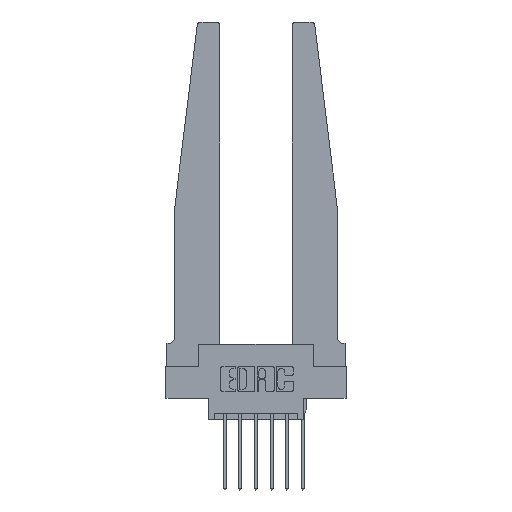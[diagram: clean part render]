
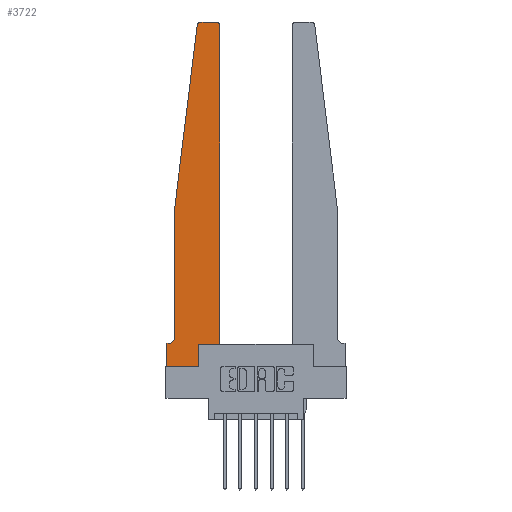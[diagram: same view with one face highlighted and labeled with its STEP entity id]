
A CAD part, top view. The second image highlights one B-rep face of the part: STEP entity #3722.
In plain terms, the highlighted planar face has unit normal (0, 0, 1).
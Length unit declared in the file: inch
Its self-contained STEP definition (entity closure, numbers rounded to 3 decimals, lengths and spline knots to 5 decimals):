
#39 = DIRECTION ( 'NONE',  ( 0., 1., 0. ) ) ;
#136 = EDGE_CURVE ( 'NONE', #623, #9087, #9557, .T. ) ;
#144 = CARTESIAN_POINT ( 'NONE',  ( 0.24675, 2.72367, 0.37 ) ) ;
#162 = VECTOR ( 'NONE', #1716, 39.37008 ) ;
#207 = VECTOR ( 'NONE', #12108, 39.37008 ) ;
#254 = ORIENTED_EDGE ( 'NONE', *, *, #5179, .T. ) ;
#458 = ORIENTED_EDGE ( 'NONE', *, *, #8291, .T. ) ;
#574 = CARTESIAN_POINT ( 'NONE',  ( 0.065, 0.1875, 0.37 ) ) ;
#623 = VERTEX_POINT ( 'NONE', #9569 ) ;
#667 = CARTESIAN_POINT ( 'NONE',  ( 0.425, 0.18, 0.37 ) ) ;
#801 = CARTESIAN_POINT ( 'NONE',  ( 0.065, 1.25, 0.37 ) ) ;
#825 = DIRECTION ( 'NONE',  ( -0.122, -0.992, 0. ) ) ;
#870 = VERTEX_POINT ( 'NONE', #7505 ) ;
#962 = VERTEX_POINT ( 'NONE', #6687 ) ;
#1385 = VECTOR ( 'NONE', #11388, 39.37008 ) ;
#1552 = VERTEX_POINT ( 'NONE', #5206 ) ;
#1575 = CARTESIAN_POINT ( 'NONE',  ( 0.25, 2.75, 0.37 ) ) ;
#1716 = DIRECTION ( 'NONE',  ( 1., 0., 0. ) ) ;
#1934 = LINE ( 'NONE', #9329, #2106 ) ;
#2003 = CIRCLE ( 'NONE', #2866, 0.03 ) ;
#2106 = VECTOR ( 'NONE', #825, 39.37008 ) ;
#2564 = VECTOR ( 'NONE', #4775, 39.37008 ) ;
#2747 = DIRECTION ( 'NONE',  ( 0., 1., 0. ) ) ;
#2781 = AXIS2_PLACEMENT_3D ( 'NONE', #12339, #7245, #10141 ) ;
#2866 = AXIS2_PLACEMENT_3D ( 'NONE', #13142, #8946, #3664 ) ;
#3076 = LINE ( 'NONE', #6185, #162 ) ;
#3124 = CARTESIAN_POINT ( 'NONE',  ( 0.2605, 0.18, 0.37 ) ) ;
#3157 = VERTEX_POINT ( 'NONE', #144 ) ;
#3275 = ORIENTED_EDGE ( 'NONE', *, *, #11091, .T. ) ;
#3395 = VERTEX_POINT ( 'NONE', #9115 ) ;
#3466 = VERTEX_POINT ( 'NONE', #13535 ) ;
#3613 = DIRECTION ( 'NONE',  ( 1., 0., 0. ) ) ;
#3664 = DIRECTION ( 'NONE',  ( 1., 0., 0. ) ) ;
#3722 = ADVANCED_FACE ( 'NONE', ( #5552 ), #6763, .T. ) ;
#3749 = LINE ( 'NONE', #1575, #207 ) ;
#3844 = ORIENTED_EDGE ( 'NONE', *, *, #9715, .T. ) ;
#3959 = ORIENTED_EDGE ( 'NONE', *, *, #136, .T. ) ;
#4170 = ORIENTED_EDGE ( 'NONE', *, *, #6065, .T. ) ;
#4281 = CARTESIAN_POINT ( 'NONE',  ( 0., 0., 0.37 ) ) ;
#4596 = VECTOR ( 'NONE', #39, 39.37008 ) ;
#4775 = DIRECTION ( 'NONE',  ( -1., 0., 0. ) ) ;
#4796 = VERTEX_POINT ( 'NONE', #13323 ) ;
#5005 = DIRECTION ( 'NONE',  ( 0., -1., 0. ) ) ;
#5108 = EDGE_CURVE ( 'NONE', #3466, #10451, #3076, .T. ) ;
#5126 = EDGE_CURVE ( 'NONE', #962, #3395, #13591, .T. ) ;
#5179 = EDGE_CURVE ( 'NONE', #870, #1552, #8766, .T. ) ;
#5206 = CARTESIAN_POINT ( 'NONE',  ( 0.395, 2.75, 0.37 ) ) ;
#5508 = CARTESIAN_POINT ( 'NONE',  ( 0.425, 0.18, 0.37 ) ) ;
#5552 = FACE_OUTER_BOUND ( 'NONE', #10927, .T. ) ;
#5947 = VECTOR ( 'NONE', #11694, 39.37008 ) ;
#6065 = EDGE_CURVE ( 'NONE', #3395, #11338, #9866, .T. ) ;
#6103 = VECTOR ( 'NONE', #5005, 39.37008 ) ;
#6185 = CARTESIAN_POINT ( 'NONE',  ( 0.425, 0.18, 0.37 ) ) ;
#6453 = CARTESIAN_POINT ( 'NONE',  ( 0.015, 0.1875, 0.37 ) ) ;
#6575 = EDGE_CURVE ( 'NONE', #11338, #623, #6877, .T. ) ;
#6599 = ORIENTED_EDGE ( 'NONE', *, *, #6575, .T. ) ;
#6687 = CARTESIAN_POINT ( 'NONE',  ( 0.065, 1.25, 0.37 ) ) ;
#6760 = DIRECTION ( 'NONE',  ( -1., 0., 0. ) ) ;
#6763 = PLANE ( 'NONE',  #11525 ) ;
#6877 = LINE ( 'NONE', #574, #2564 ) ;
#6888 = VERTEX_POINT ( 'NONE', #11595 ) ;
#6959 = LINE ( 'NONE', #667, #4596 ) ;
#7245 = DIRECTION ( 'NONE',  ( 0., 0., 1. ) ) ;
#7371 = LINE ( 'NONE', #3124, #7919 ) ;
#7505 = CARTESIAN_POINT ( 'NONE',  ( 0.425, 2.72, 0.37 ) ) ;
#7919 = VECTOR ( 'NONE', #2747, 39.37008 ) ;
#7932 = CARTESIAN_POINT ( 'NONE',  ( 0.015, 0.2375, 0.37 ) ) ;
#8291 = EDGE_CURVE ( 'NONE', #4796, #3466, #7371, .T. ) ;
#8465 = ORIENTED_EDGE ( 'NONE', *, *, #9701, .T. ) ;
#8557 = ORIENTED_EDGE ( 'NONE', *, *, #5126, .T. ) ;
#8766 = CIRCLE ( 'NONE', #2781, 0.03 ) ;
#8835 = DIRECTION ( 'NONE',  ( 0., 0., -1. ) ) ;
#8839 = CARTESIAN_POINT ( 'NONE',  ( 0., 0.1875, 0.37 ) ) ;
#8946 = DIRECTION ( 'NONE',  ( 0., 0., 1. ) ) ;
#9087 = VERTEX_POINT ( 'NONE', #10060 ) ;
#9115 = CARTESIAN_POINT ( 'NONE',  ( 0.065, 0.2375, 0.37 ) ) ;
#9329 = CARTESIAN_POINT ( 'NONE',  ( 0.065, 1.25, 0.37 ) ) ;
#9557 = LINE ( 'NONE', #4281, #1385 ) ;
#9569 = CARTESIAN_POINT ( 'NONE',  ( 0., 0.1875, 0.37 ) ) ;
#9701 = EDGE_CURVE ( 'NONE', #1552, #6888, #3749, .T. ) ;
#9715 = EDGE_CURVE ( 'NONE', #10451, #870, #6959, .T. ) ;
#9866 = CIRCLE ( 'NONE', #12920, 0.05 ) ;
#10060 = CARTESIAN_POINT ( 'NONE',  ( 0., 0., 0.37 ) ) ;
#10141 = DIRECTION ( 'NONE',  ( 1., 0., 0. ) ) ;
#10451 = VERTEX_POINT ( 'NONE', #5508 ) ;
#10552 = ORIENTED_EDGE ( 'NONE', *, *, #13194, .T. ) ;
#10803 = EDGE_CURVE ( 'NONE', #9087, #4796, #12457, .T. ) ;
#10927 = EDGE_LOOP ( 'NONE', ( #8465, #3275, #10552, #8557, #4170, #6599, #3959, #13222, #458, #12859, #3844, #254 ) ) ;
#11091 = EDGE_CURVE ( 'NONE', #6888, #3157, #2003, .T. ) ;
#11338 = VERTEX_POINT ( 'NONE', #6453 ) ;
#11388 = DIRECTION ( 'NONE',  ( 0., -1., 0. ) ) ;
#11525 = AXIS2_PLACEMENT_3D ( 'NONE', #8839, #13087, #3613 ) ;
#11595 = CARTESIAN_POINT ( 'NONE',  ( 0.27653, 2.75, 0.37 ) ) ;
#11694 = DIRECTION ( 'NONE',  ( 1., 0., 0. ) ) ;
#12108 = DIRECTION ( 'NONE',  ( -1., 0., 0. ) ) ;
#12339 = CARTESIAN_POINT ( 'NONE',  ( 0.395, 2.72, 0.37 ) ) ;
#12457 = LINE ( 'NONE', #13519, #5947 ) ;
#12859 = ORIENTED_EDGE ( 'NONE', *, *, #5108, .T. ) ;
#12920 = AXIS2_PLACEMENT_3D ( 'NONE', #7932, #8835, #6760 ) ;
#13087 = DIRECTION ( 'NONE',  ( 0., 0., 1. ) ) ;
#13142 = CARTESIAN_POINT ( 'NONE',  ( 0.27653, 2.72, 0.37 ) ) ;
#13194 = EDGE_CURVE ( 'NONE', #3157, #962, #1934, .T. ) ;
#13222 = ORIENTED_EDGE ( 'NONE', *, *, #10803, .T. ) ;
#13323 = CARTESIAN_POINT ( 'NONE',  ( 0.2605, 0., 0.37 ) ) ;
#13519 = CARTESIAN_POINT ( 'NONE',  ( 0., 0., 0.37 ) ) ;
#13535 = CARTESIAN_POINT ( 'NONE',  ( 0.2605, 0.18, 0.37 ) ) ;
#13591 = LINE ( 'NONE', #801, #6103 ) ;
